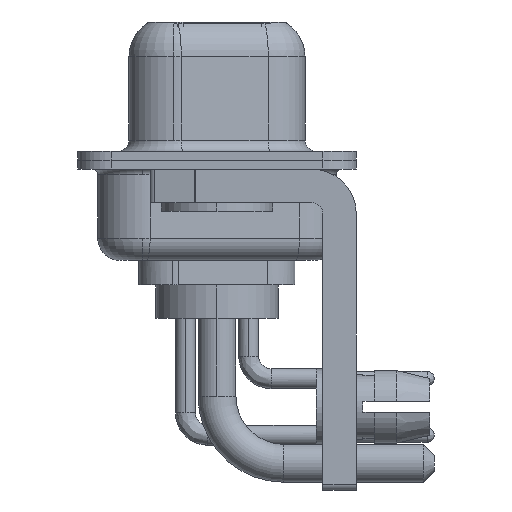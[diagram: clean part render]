
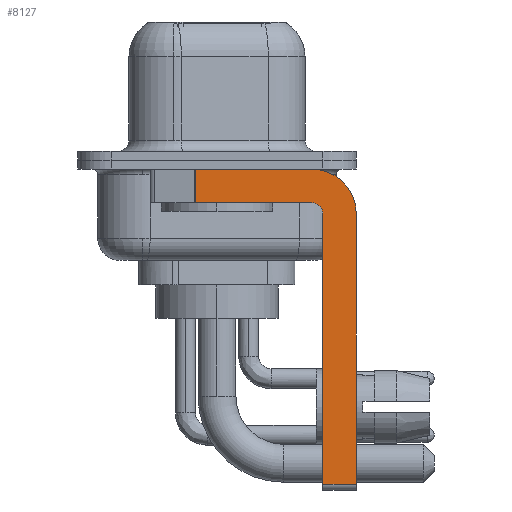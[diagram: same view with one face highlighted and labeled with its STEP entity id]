
A CAD part, left-side view. The second image highlights one B-rep face of the part: STEP entity #8127.
In plain terms, the highlighted planar face has unit normal (-1, 0, 0).
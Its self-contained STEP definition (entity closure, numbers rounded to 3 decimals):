
#21 = DIRECTION ( 'NONE',  ( 1., 0., 0. ) ) ;
#730 = DIRECTION ( 'NONE',  ( 0., 0., -1. ) ) ;
#739 = EDGE_CURVE ( 'NONE', #13653, #4030, #7476, .T. ) ;
#985 = DIRECTION ( 'NONE',  ( 1., 0., 0. ) ) ;
#1142 = DIRECTION ( 'NONE',  ( 0., -1., 0. ) ) ;
#1239 = PLANE ( 'NONE',  #17811 ) ;
#1865 = VERTEX_POINT ( 'NONE', #15642 ) ;
#1901 = CARTESIAN_POINT ( 'NONE',  ( -2.9, -4.25, -1.9 ) ) ;
#2208 = ORIENTED_EDGE ( 'NONE', *, *, #19318, .F. ) ;
#2521 = FACE_OUTER_BOUND ( 'NONE', #19031, .T. ) ;
#2825 = CARTESIAN_POINT ( 'NONE',  ( -2.9, -4.25, -2.4 ) ) ;
#3127 = EDGE_CURVE ( 'NONE', #3879, #15836, #19283, .T. ) ;
#3149 = LINE ( 'NONE', #9399, #7190 ) ;
#3470 = CARTESIAN_POINT ( 'NONE',  ( -2.9, -4.75, -14.55 ) ) ;
#3833 = VERTEX_POINT ( 'NONE', #8362 ) ;
#3879 = VERTEX_POINT ( 'NONE', #11356 ) ;
#4030 = VERTEX_POINT ( 'NONE', #1901 ) ;
#4246 = ORIENTED_EDGE ( 'NONE', *, *, #5526, .T. ) ;
#4720 = DIRECTION ( 'NONE',  ( 0., -1., 0. ) ) ;
#5109 = ORIENTED_EDGE ( 'NONE', *, *, #3127, .F. ) ;
#5412 = EDGE_CURVE ( 'NONE', #12666, #13653, #8063, .T. ) ;
#5526 = EDGE_CURVE ( 'NONE', #3833, #13591, #9767, .T. ) ;
#5536 = ORIENTED_EDGE ( 'NONE', *, *, #19587, .T. ) ;
#5644 = EDGE_CURVE ( 'NONE', #4030, #13591, #16608, .T. ) ;
#5736 = DIRECTION ( 'NONE',  ( 0., 0., -1. ) ) ;
#6568 = CARTESIAN_POINT ( 'NONE',  ( -2.9, -4.75, -14.8 ) ) ;
#6653 = ORIENTED_EDGE ( 'NONE', *, *, #5412, .F. ) ;
#6717 = LINE ( 'NONE', #15678, #10684 ) ;
#6886 = AXIS2_PLACEMENT_3D ( 'NONE', #10432, #985, #5736 ) ;
#7190 = VECTOR ( 'NONE', #4720, 1000. ) ;
#7291 = DIRECTION ( 'NONE',  ( 0., 0., -1. ) ) ;
#7476 = CIRCLE ( 'NONE', #11308, 0.5 ) ;
#7574 = VECTOR ( 'NONE', #730, 1000. ) ;
#8063 = LINE ( 'NONE', #6568, #13915 ) ;
#8127 = ADVANCED_FACE ( 'NONE', ( #2521 ), #1239, .F. ) ;
#8266 = CARTESIAN_POINT ( 'NONE',  ( -2.9, 0.978, -1.9 ) ) ;
#8362 = CARTESIAN_POINT ( 'NONE',  ( -2.9, 0.978, -0.4 ) ) ;
#9399 = CARTESIAN_POINT ( 'NONE',  ( -2.9, -4.25, -14.55 ) ) ;
#9651 = CARTESIAN_POINT ( 'NONE',  ( -2.9, -6.25, -2.4 ) ) ;
#9767 = LINE ( 'NONE', #8266, #7574 ) ;
#10191 = CARTESIAN_POINT ( 'NONE',  ( -2.9, 3., -0.4 ) ) ;
#10432 = CARTESIAN_POINT ( 'NONE',  ( -2.9, -4.25, -2.4 ) ) ;
#10684 = VECTOR ( 'NONE', #12805, 1000. ) ;
#10755 = VECTOR ( 'NONE', #12048, 1000. ) ;
#11308 = AXIS2_PLACEMENT_3D ( 'NONE', #13014, #14588, #11526 ) ;
#11356 = CARTESIAN_POINT ( 'NONE',  ( -2.9, -4.25, -0.4 ) ) ;
#11526 = DIRECTION ( 'NONE',  ( 0., 0., 1. ) ) ;
#12048 = DIRECTION ( 'NONE',  ( 0., 1., 0. ) ) ;
#12586 = CARTESIAN_POINT ( 'NONE',  ( -2.9, 0.978, -1.9 ) ) ;
#12666 = VERTEX_POINT ( 'NONE', #3470 ) ;
#12805 = DIRECTION ( 'NONE',  ( 0., 0., -1. ) ) ;
#13014 = CARTESIAN_POINT ( 'NONE',  ( -2.9, -4.25, -2.4 ) ) ;
#13144 = ORIENTED_EDGE ( 'NONE', *, *, #5644, .F. ) ;
#13591 = VERTEX_POINT ( 'NONE', #12586 ) ;
#13653 = VERTEX_POINT ( 'NONE', #18417 ) ;
#13872 = EDGE_CURVE ( 'NONE', #3833, #3879, #19226, .T. ) ;
#13915 = VECTOR ( 'NONE', #15231, 1000. ) ;
#13965 = ORIENTED_EDGE ( 'NONE', *, *, #13872, .F. ) ;
#13999 = VECTOR ( 'NONE', #1142, 1000. ) ;
#14588 = DIRECTION ( 'NONE',  ( -1., 0., 0. ) ) ;
#14834 = CARTESIAN_POINT ( 'NONE',  ( -2.9, -4.25, -1.9 ) ) ;
#15231 = DIRECTION ( 'NONE',  ( 0., 0., 1. ) ) ;
#15642 = CARTESIAN_POINT ( 'NONE',  ( -2.9, -6.25, -14.55 ) ) ;
#15678 = CARTESIAN_POINT ( 'NONE',  ( -2.9, -6.25, -2.4 ) ) ;
#15836 = VERTEX_POINT ( 'NONE', #9651 ) ;
#16608 = LINE ( 'NONE', #14834, #10755 ) ;
#17336 = ORIENTED_EDGE ( 'NONE', *, *, #739, .F. ) ;
#17811 = AXIS2_PLACEMENT_3D ( 'NONE', #2825, #21, #7291 ) ;
#18417 = CARTESIAN_POINT ( 'NONE',  ( -2.9, -4.75, -2.4 ) ) ;
#19031 = EDGE_LOOP ( 'NONE', ( #13965, #4246, #13144, #17336, #6653, #5536, #2208, #5109 ) ) ;
#19226 = LINE ( 'NONE', #10191, #13999 ) ;
#19283 = CIRCLE ( 'NONE', #6886, 2. ) ;
#19318 = EDGE_CURVE ( 'NONE', #15836, #1865, #6717, .T. ) ;
#19587 = EDGE_CURVE ( 'NONE', #12666, #1865, #3149, .T. ) ;
